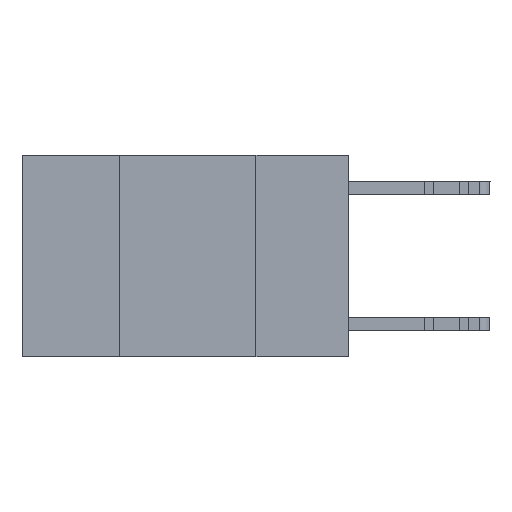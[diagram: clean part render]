
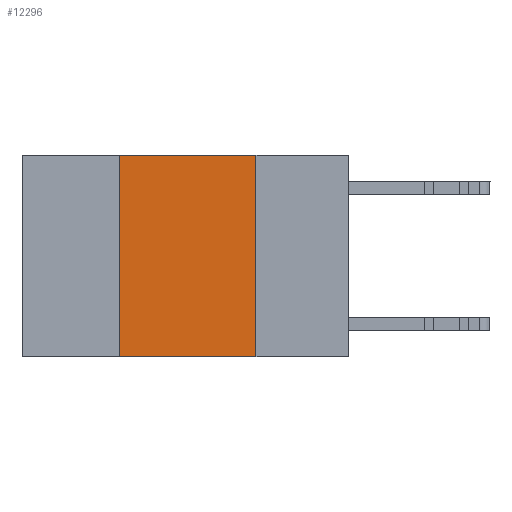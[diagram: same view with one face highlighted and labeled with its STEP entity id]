
A CAD part, left-side view. The second image highlights one B-rep face of the part: STEP entity #12296.
In plain terms, the highlighted planar face has unit normal (-1, 0, 0).
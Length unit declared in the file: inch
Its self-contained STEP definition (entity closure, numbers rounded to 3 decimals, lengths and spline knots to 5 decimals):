
#84 = EDGE_CURVE ( 'NONE', #12089, #11610, #3090, .T. ) ;
#1056 = DIRECTION ( 'NONE',  ( 0., -1., 0. ) ) ;
#1385 = EDGE_CURVE ( 'NONE', #4264, #12484, #8350, .T. ) ;
#1479 = VECTOR ( 'NONE', #12494, 39.37008 ) ;
#2799 = LINE ( 'NONE', #14200, #3919 ) ;
#3090 = LINE ( 'NONE', #14204, #1479 ) ;
#3108 = CARTESIAN_POINT ( 'NONE',  ( 0., 0.6, 0. ) ) ;
#3284 = ORIENTED_EDGE ( 'NONE', *, *, #16708, .F. ) ;
#3919 = VECTOR ( 'NONE', #21296, 39.37008 ) ;
#4264 = VERTEX_POINT ( 'NONE', #6682 ) ;
#6350 = EDGE_LOOP ( 'NONE', ( #15051, #11014, #3284, #13659 ) ) ;
#6396 = VECTOR ( 'NONE', #9019, 39.37008 ) ;
#6682 = CARTESIAN_POINT ( 'NONE',  ( 0., 0.42, 0. ) ) ;
#8350 = LINE ( 'NONE', #14828, #18535 ) ;
#8473 = DIRECTION ( 'NONE',  ( 0., 0., -1. ) ) ;
#9019 = DIRECTION ( 'NONE',  ( 0., 0., 1. ) ) ;
#9180 = CARTESIAN_POINT ( 'NONE',  ( 0., 0.42, 0. ) ) ;
#10201 = DIRECTION ( 'NONE',  ( 1., 0., 0. ) ) ;
#10923 = PLANE ( 'NONE',  #18536 ) ;
#11014 = ORIENTED_EDGE ( 'NONE', *, *, #1385, .F. ) ;
#11610 = VERTEX_POINT ( 'NONE', #30015 ) ;
#12089 = VERTEX_POINT ( 'NONE', #22862 ) ;
#12296 = ADVANCED_FACE ( 'NONE', ( #22947 ), #10923, .F. ) ;
#12484 = VERTEX_POINT ( 'NONE', #27738 ) ;
#12494 = DIRECTION ( 'NONE',  ( 0., -1., 0. ) ) ;
#13659 = ORIENTED_EDGE ( 'NONE', *, *, #84, .T. ) ;
#14200 = CARTESIAN_POINT ( 'NONE',  ( 0., 0.17, 0. ) ) ;
#14204 = CARTESIAN_POINT ( 'NONE',  ( 0., 0.6, -0.37 ) ) ;
#14828 = CARTESIAN_POINT ( 'NONE',  ( 0., 0.6, 0. ) ) ;
#15051 = ORIENTED_EDGE ( 'NONE', *, *, #18414, .F. ) ;
#16708 = EDGE_CURVE ( 'NONE', #12089, #4264, #25199, .T. ) ;
#18414 = EDGE_CURVE ( 'NONE', #12484, #11610, #2799, .T. ) ;
#18535 = VECTOR ( 'NONE', #1056, 39.37008 ) ;
#18536 = AXIS2_PLACEMENT_3D ( 'NONE', #3108, #10201, #8473 ) ;
#21296 = DIRECTION ( 'NONE',  ( 0., 0., -1. ) ) ;
#22862 = CARTESIAN_POINT ( 'NONE',  ( 0., 0.42, -0.37 ) ) ;
#22947 = FACE_OUTER_BOUND ( 'NONE', #6350, .T. ) ;
#25199 = LINE ( 'NONE', #9180, #6396 ) ;
#27738 = CARTESIAN_POINT ( 'NONE',  ( 0., 0.17, 0. ) ) ;
#30015 = CARTESIAN_POINT ( 'NONE',  ( 0., 0.17, -0.37 ) ) ;
